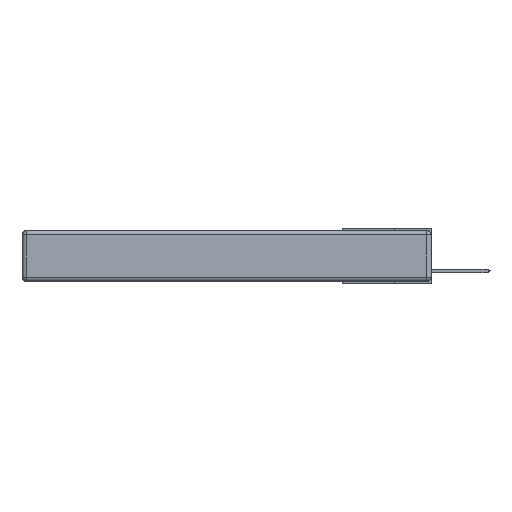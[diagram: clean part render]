
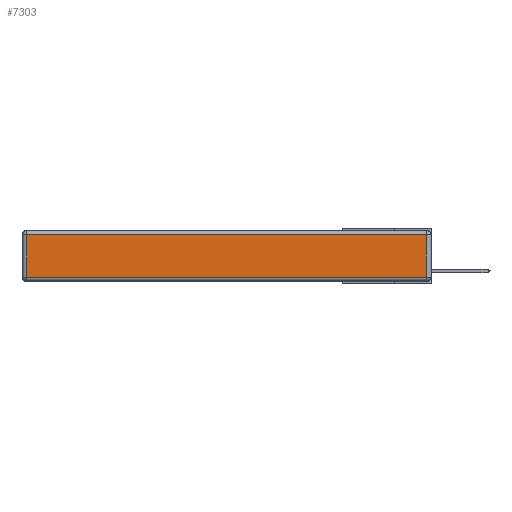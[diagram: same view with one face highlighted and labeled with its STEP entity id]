
A CAD part, left-side view. The second image highlights one B-rep face of the part: STEP entity #7303.
In plain terms, the highlighted planar face has unit normal (-1, 0, 0).
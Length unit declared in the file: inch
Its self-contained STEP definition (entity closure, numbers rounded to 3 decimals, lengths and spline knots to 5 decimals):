
#268 = EDGE_CURVE ( 'NONE', #18487, #23472, #23767, .T. ) ;
#592 = ORIENTED_EDGE ( 'NONE', *, *, #18963, .T. ) ;
#948 = VECTOR ( 'NONE', #20748, 39.37008 ) ;
#1755 = CARTESIAN_POINT ( 'NONE',  ( 0., 0., -0.313 ) ) ;
#2501 = CARTESIAN_POINT ( 'NONE',  ( 0., 2.75, -0.03 ) ) ;
#2697 = DIRECTION ( 'NONE',  ( 0., 1., 0. ) ) ;
#4673 = VECTOR ( 'NONE', #24499, 39.37008 ) ;
#5877 = LINE ( 'NONE', #2501, #19095 ) ;
#6610 = CARTESIAN_POINT ( 'NONE',  ( 0., 0.03, -0.313 ) ) ;
#6892 = EDGE_LOOP ( 'NONE', ( #21514, #13760, #592, #22984 ) ) ;
#7303 = ADVANCED_FACE ( 'NONE', ( #19213 ), #14595, .T. ) ;
#8349 = CARTESIAN_POINT ( 'NONE',  ( 0., 2.72, -0.03 ) ) ;
#12589 = CARTESIAN_POINT ( 'NONE',  ( 0., 0.03, -0.343 ) ) ;
#12683 = LINE ( 'NONE', #12589, #13341 ) ;
#12789 = CARTESIAN_POINT ( 'NONE',  ( 0., 2.72, -0.313 ) ) ;
#12994 = VERTEX_POINT ( 'NONE', #23777 ) ;
#13341 = VECTOR ( 'NONE', #21235, 39.37008 ) ;
#13760 = ORIENTED_EDGE ( 'NONE', *, *, #14427, .T. ) ;
#14427 = EDGE_CURVE ( 'NONE', #23472, #12994, #12683, .T. ) ;
#14595 = PLANE ( 'NONE',  #27256 ) ;
#17728 = VERTEX_POINT ( 'NONE', #8349 ) ;
#18487 = VERTEX_POINT ( 'NONE', #12789 ) ;
#18963 = EDGE_CURVE ( 'NONE', #12994, #17728, #5877, .T. ) ;
#19031 = CARTESIAN_POINT ( 'NONE',  ( 0., 0., -0.343 ) ) ;
#19095 = VECTOR ( 'NONE', #2697, 39.37008 ) ;
#19213 = FACE_OUTER_BOUND ( 'NONE', #6892, .T. ) ;
#19879 = EDGE_CURVE ( 'NONE', #17728, #18487, #24927, .T. ) ;
#20748 = DIRECTION ( 'NONE',  ( 0., 0., -1. ) ) ;
#20844 = CARTESIAN_POINT ( 'NONE',  ( 0., 2.72, -0.343 ) ) ;
#21153 = DIRECTION ( 'NONE',  ( -1., 0., 0. ) ) ;
#21235 = DIRECTION ( 'NONE',  ( 0., 0., 1. ) ) ;
#21514 = ORIENTED_EDGE ( 'NONE', *, *, #268, .T. ) ;
#22984 = ORIENTED_EDGE ( 'NONE', *, *, #19879, .T. ) ;
#23472 = VERTEX_POINT ( 'NONE', #6610 ) ;
#23767 = LINE ( 'NONE', #1755, #4673 ) ;
#23777 = CARTESIAN_POINT ( 'NONE',  ( 0., 0.03, -0.03 ) ) ;
#24499 = DIRECTION ( 'NONE',  ( 0., -1., 0. ) ) ;
#24927 = LINE ( 'NONE', #20844, #948 ) ;
#25340 = DIRECTION ( 'NONE',  ( 0., 0., 1. ) ) ;
#27256 = AXIS2_PLACEMENT_3D ( 'NONE', #19031, #21153, #25340 ) ;
